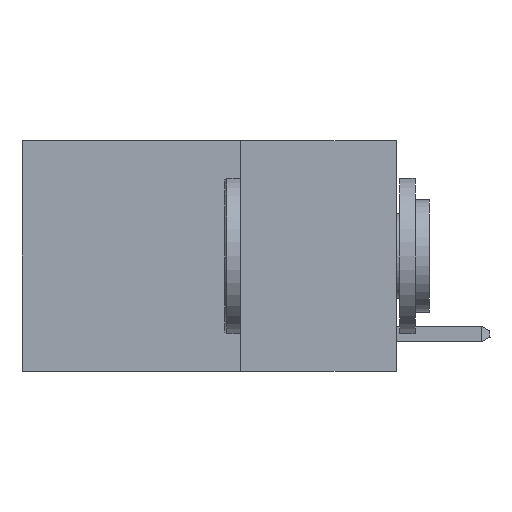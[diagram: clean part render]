
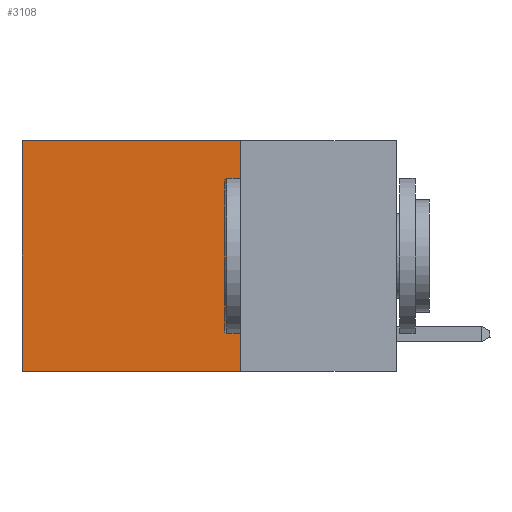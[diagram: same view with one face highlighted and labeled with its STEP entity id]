
A CAD part, left-side view. The second image highlights one B-rep face of the part: STEP entity #3108.
In plain terms, the highlighted planar face has unit normal (-1, 0, 0).
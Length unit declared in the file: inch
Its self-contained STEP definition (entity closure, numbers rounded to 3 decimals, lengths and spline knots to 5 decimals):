
#1044 = CARTESIAN_POINT ( 'NONE',  ( 0.2625, 0.6, 0. ) ) ;
#3025 = VERTEX_POINT ( 'NONE', #5054 ) ;
#3108 = ADVANCED_FACE ( 'NONE', ( #25620 ), #14333, .F. ) ;
#3720 = CARTESIAN_POINT ( 'NONE',  ( 0.2625, 0.25, 0. ) ) ;
#4408 = DIRECTION ( 'NONE',  ( 0., 0., -1. ) ) ;
#5054 = CARTESIAN_POINT ( 'NONE',  ( 0.2625, 0.6, -0.37 ) ) ;
#5588 = VECTOR ( 'NONE', #8925, 39.37008 ) ;
#5607 = DIRECTION ( 'NONE',  ( 0., 1., 0. ) ) ;
#5726 = EDGE_CURVE ( 'NONE', #5839, #3025, #18238, .T. ) ;
#5839 = VERTEX_POINT ( 'NONE', #13633 ) ;
#6645 = ORIENTED_EDGE ( 'NONE', *, *, #15002, .T. ) ;
#6648 = ORIENTED_EDGE ( 'NONE', *, *, #27311, .T. ) ;
#7039 = AXIS2_PLACEMENT_3D ( 'NONE', #14181, #9842, #14613 ) ;
#8925 = DIRECTION ( 'NONE',  ( 0., 0., -1. ) ) ;
#9061 = VERTEX_POINT ( 'NONE', #1044 ) ;
#9510 = DIRECTION ( 'NONE',  ( 0., 1., 0. ) ) ;
#9842 = DIRECTION ( 'NONE',  ( 1., 0., 0. ) ) ;
#10154 = VECTOR ( 'NONE', #5607, 39.37008 ) ;
#11046 = ORIENTED_EDGE ( 'NONE', *, *, #5726, .F. ) ;
#13633 = CARTESIAN_POINT ( 'NONE',  ( 0.2625, 0.25, -0.37 ) ) ;
#14181 = CARTESIAN_POINT ( 'NONE',  ( 0.2625, 0.25, 0. ) ) ;
#14333 = PLANE ( 'NONE',  #7039 ) ;
#14613 = DIRECTION ( 'NONE',  ( 0., 0., -1. ) ) ;
#15002 = EDGE_CURVE ( 'NONE', #18538, #9061, #23581, .T. ) ;
#15157 = LINE ( 'NONE', #23998, #24987 ) ;
#15758 = CARTESIAN_POINT ( 'NONE',  ( 0.2625, 0.25, 0. ) ) ;
#18238 = LINE ( 'NONE', #20824, #25212 ) ;
#18446 = EDGE_CURVE ( 'NONE', #18538, #5839, #22283, .T. ) ;
#18538 = VERTEX_POINT ( 'NONE', #15758 ) ;
#18633 = ORIENTED_EDGE ( 'NONE', *, *, #18446, .F. ) ;
#19071 = EDGE_LOOP ( 'NONE', ( #6648, #11046, #18633, #6645 ) ) ;
#20824 = CARTESIAN_POINT ( 'NONE',  ( 0.2625, 0.25, -0.37 ) ) ;
#22283 = LINE ( 'NONE', #24164, #5588 ) ;
#23581 = LINE ( 'NONE', #3720, #10154 ) ;
#23998 = CARTESIAN_POINT ( 'NONE',  ( 0.2625, 0.6, 0. ) ) ;
#24164 = CARTESIAN_POINT ( 'NONE',  ( 0.2625, 0.25, 0. ) ) ;
#24987 = VECTOR ( 'NONE', #4408, 39.37008 ) ;
#25212 = VECTOR ( 'NONE', #9510, 39.37008 ) ;
#25620 = FACE_OUTER_BOUND ( 'NONE', #19071, .T. ) ;
#27311 = EDGE_CURVE ( 'NONE', #9061, #3025, #15157, .T. ) ;
